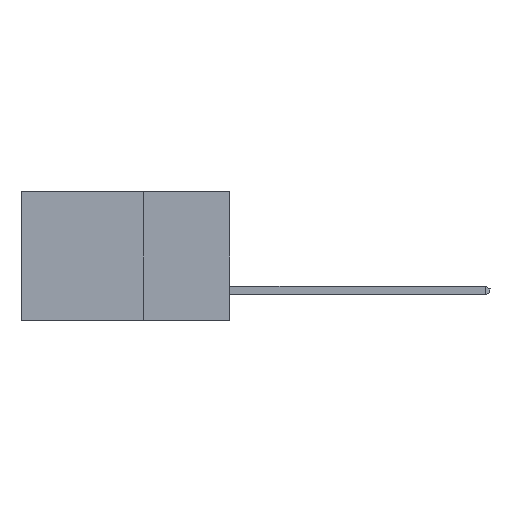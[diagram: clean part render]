
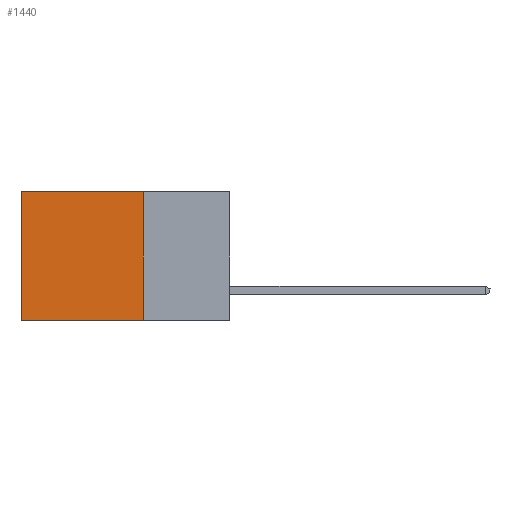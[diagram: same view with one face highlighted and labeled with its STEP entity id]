
A CAD part, left-side view. The second image highlights one B-rep face of the part: STEP entity #1440.
In plain terms, the highlighted planar face has unit normal (-1, 0, 0).
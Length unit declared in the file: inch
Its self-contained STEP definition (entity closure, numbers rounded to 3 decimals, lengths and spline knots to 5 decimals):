
#682 = CARTESIAN_POINT ( 'NONE',  ( 0.2615, 0.25, -0.37 ) ) ;
#874 = CARTESIAN_POINT ( 'NONE',  ( 0.2615, 0.6, -0.37 ) ) ;
#1440 = ADVANCED_FACE ( 'NONE', ( #1449 ), #13772, .F. ) ;
#1449 = FACE_OUTER_BOUND ( 'NONE', #15698, .T. ) ;
#1997 = LINE ( 'NONE', #682, #8570 ) ;
#2658 = ORIENTED_EDGE ( 'NONE', *, *, #14101, .F. ) ;
#3016 = VECTOR ( 'NONE', #8411, 39.37008 ) ;
#3393 = CARTESIAN_POINT ( 'NONE',  ( 0.2615, 0.25, 0. ) ) ;
#4075 = VERTEX_POINT ( 'NONE', #874 ) ;
#4421 = CARTESIAN_POINT ( 'NONE',  ( 0.2615, 0.6, 0. ) ) ;
#4939 = LINE ( 'NONE', #3393, #3016 ) ;
#7318 = LINE ( 'NONE', #12462, #15724 ) ;
#7561 = CARTESIAN_POINT ( 'NONE',  ( 0.2615, 0.25, -0.37 ) ) ;
#7850 = EDGE_CURVE ( 'NONE', #15240, #4075, #8440, .T. ) ;
#8411 = DIRECTION ( 'NONE',  ( 0., 1., 0. ) ) ;
#8433 = VERTEX_POINT ( 'NONE', #15242 ) ;
#8440 = LINE ( 'NONE', #15090, #15162 ) ;
#8570 = VECTOR ( 'NONE', #12093, 39.37008 ) ;
#9933 = AXIS2_PLACEMENT_3D ( 'NONE', #7561, #14029, #11445 ) ;
#10201 = VERTEX_POINT ( 'NONE', #13214 ) ;
#10546 = ORIENTED_EDGE ( 'NONE', *, *, #13811, .T. ) ;
#10590 = EDGE_CURVE ( 'NONE', #10201, #8433, #1997, .T. ) ;
#11025 = DIRECTION ( 'NONE',  ( 0., 0., -1. ) ) ;
#11241 = ORIENTED_EDGE ( 'NONE', *, *, #10590, .F. ) ;
#11445 = DIRECTION ( 'NONE',  ( 0., 0., -1. ) ) ;
#11843 = ORIENTED_EDGE ( 'NONE', *, *, #7850, .T. ) ;
#12093 = DIRECTION ( 'NONE',  ( 0., 0., -1. ) ) ;
#12462 = CARTESIAN_POINT ( 'NONE',  ( 0.2615, 0.25, -0.37 ) ) ;
#13214 = CARTESIAN_POINT ( 'NONE',  ( 0.2615, 0.25, 0. ) ) ;
#13772 = PLANE ( 'NONE',  #9933 ) ;
#13811 = EDGE_CURVE ( 'NONE', #10201, #15240, #4939, .T. ) ;
#14029 = DIRECTION ( 'NONE',  ( 1., 0., 0. ) ) ;
#14101 = EDGE_CURVE ( 'NONE', #8433, #4075, #7318, .T. ) ;
#15090 = CARTESIAN_POINT ( 'NONE',  ( 0.2615, 0.6, -0.37 ) ) ;
#15162 = VECTOR ( 'NONE', #11025, 39.37008 ) ;
#15240 = VERTEX_POINT ( 'NONE', #4421 ) ;
#15242 = CARTESIAN_POINT ( 'NONE',  ( 0.2615, 0.25, -0.37 ) ) ;
#15698 = EDGE_LOOP ( 'NONE', ( #11843, #2658, #11241, #10546 ) ) ;
#15724 = VECTOR ( 'NONE', #16283, 39.37008 ) ;
#16283 = DIRECTION ( 'NONE',  ( 0., 1., 0. ) ) ;
